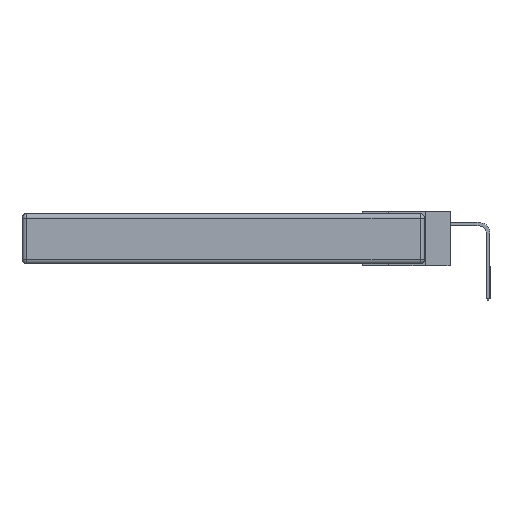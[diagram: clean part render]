
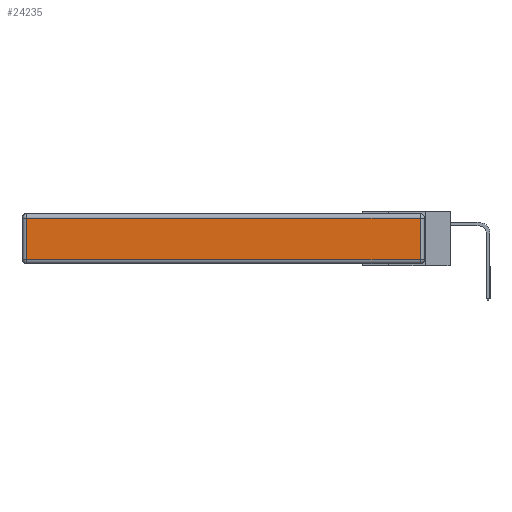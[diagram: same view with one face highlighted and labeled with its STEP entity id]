
A CAD part, left-side view. The second image highlights one B-rep face of the part: STEP entity #24235.
In plain terms, the highlighted planar face has unit normal (-1, 0, 0).
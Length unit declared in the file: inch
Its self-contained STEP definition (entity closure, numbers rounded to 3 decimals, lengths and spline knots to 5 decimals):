
#1425 = EDGE_CURVE ( 'NONE', #2003, #9336, #32674, .T. ) ;
#1428 = DIRECTION ( 'NONE',  ( 0., -1., 0. ) ) ;
#1943 = CARTESIAN_POINT ( 'NONE',  ( 0., 2.75, -0.03 ) ) ;
#2003 = VERTEX_POINT ( 'NONE', #32543 ) ;
#2024 = CARTESIAN_POINT ( 'NONE',  ( 0., 0.03, -0.343 ) ) ;
#3999 = EDGE_LOOP ( 'NONE', ( #15712, #21064, #4759, #6686 ) ) ;
#4759 = ORIENTED_EDGE ( 'NONE', *, *, #1425, .T. ) ;
#6607 = EDGE_CURVE ( 'NONE', #9336, #18565, #24506, .T. ) ;
#6686 = ORIENTED_EDGE ( 'NONE', *, *, #6607, .T. ) ;
#6857 = EDGE_CURVE ( 'NONE', #18565, #8411, #30995, .T. ) ;
#8310 = CARTESIAN_POINT ( 'NONE',  ( 0., 2.72, -0.03 ) ) ;
#8411 = VERTEX_POINT ( 'NONE', #31572 ) ;
#9336 = VERTEX_POINT ( 'NONE', #8310 ) ;
#9399 = CARTESIAN_POINT ( 'NONE',  ( 0., 0., -0.313 ) ) ;
#10792 = VECTOR ( 'NONE', #22583, 39.37008 ) ;
#11348 = CARTESIAN_POINT ( 'NONE',  ( 0., 2.72, -0.343 ) ) ;
#11496 = LINE ( 'NONE', #2024, #31348 ) ;
#11979 = DIRECTION ( 'NONE',  ( 0., 0., 1. ) ) ;
#12139 = AXIS2_PLACEMENT_3D ( 'NONE', #22531, #19603, #11979 ) ;
#13494 = CARTESIAN_POINT ( 'NONE',  ( 0., 2.72, -0.313 ) ) ;
#13934 = FACE_OUTER_BOUND ( 'NONE', #3999, .T. ) ;
#15712 = ORIENTED_EDGE ( 'NONE', *, *, #6857, .T. ) ;
#18565 = VERTEX_POINT ( 'NONE', #13494 ) ;
#19603 = DIRECTION ( 'NONE',  ( -1., 0., 0. ) ) ;
#20175 = DIRECTION ( 'NONE',  ( 0., 0., 1. ) ) ;
#21064 = ORIENTED_EDGE ( 'NONE', *, *, #27642, .T. ) ;
#22304 = PLANE ( 'NONE',  #12139 ) ;
#22531 = CARTESIAN_POINT ( 'NONE',  ( 0., 0., -0.343 ) ) ;
#22583 = DIRECTION ( 'NONE',  ( 0., 1., 0. ) ) ;
#24235 = ADVANCED_FACE ( 'NONE', ( #13934 ), #22304, .T. ) ;
#24506 = LINE ( 'NONE', #11348, #25747 ) ;
#25747 = VECTOR ( 'NONE', #29219, 39.37008 ) ;
#27642 = EDGE_CURVE ( 'NONE', #8411, #2003, #11496, .T. ) ;
#29219 = DIRECTION ( 'NONE',  ( 0., 0., -1. ) ) ;
#30995 = LINE ( 'NONE', #9399, #32647 ) ;
#31348 = VECTOR ( 'NONE', #20175, 39.37008 ) ;
#31572 = CARTESIAN_POINT ( 'NONE',  ( 0., 0.03, -0.313 ) ) ;
#32543 = CARTESIAN_POINT ( 'NONE',  ( 0., 0.03, -0.03 ) ) ;
#32647 = VECTOR ( 'NONE', #1428, 39.37008 ) ;
#32674 = LINE ( 'NONE', #1943, #10792 ) ;
